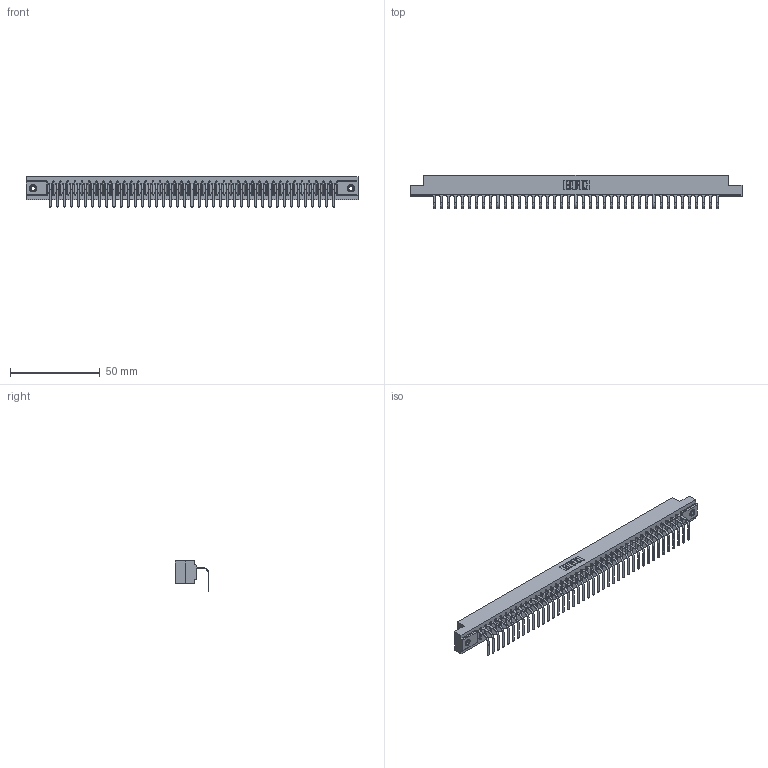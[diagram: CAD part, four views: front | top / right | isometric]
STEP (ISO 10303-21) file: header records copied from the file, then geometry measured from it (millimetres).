
FILE_DESCRIPTION (( 'STEP AP203' ), '1' );
FILE_NAME ('357-041-558-108.STEP', '2022-07-13T18:16:51', ( '' ), ( '' ), 'SwSTEP 2.0', 'SolidWorks 2020', '' );
FILE_SCHEMA (( 'CONFIG_CONTROL_DESIGN' ));
Length unit declared in the file: inch
Products named in the file (4): 345-250-001_345-250-003-102; 357-041-558-108; 307 Part_.156 Dia Mounting Holes; 307-290-001_558 - 2 (Single)
Assembly tree (44 placements, depth 2):
  357-041-558-108
    307 Part_.156 Dia Mounting Holes
    307-290-001_558 - 2 (Single)  x41
    345-250-001_345-250-003-102  x2
Bounding box: 185.47 x 18.78 x 16.8 mm (x, y, z)
Volume: 19410.8 mm3; surface area: 21656.5 mm2
Topology: 44 solids, 44 shells, 2680 faces, 7593 edges, 4886 vertices
Faces by surface type: plane 1701, cylinder 879, sphere 84, cone 12, torus 4
Entity records: 36561 total; most frequent: CARTESIAN_POINT 6139, ORIENTED_EDGE 6118, DIRECTION 5981, EDGE_CURVE 3059, VECTOR 2345, LINE 2345, VERTEX_POINT 1976, AXIS2_PLACEMENT_3D 1818
